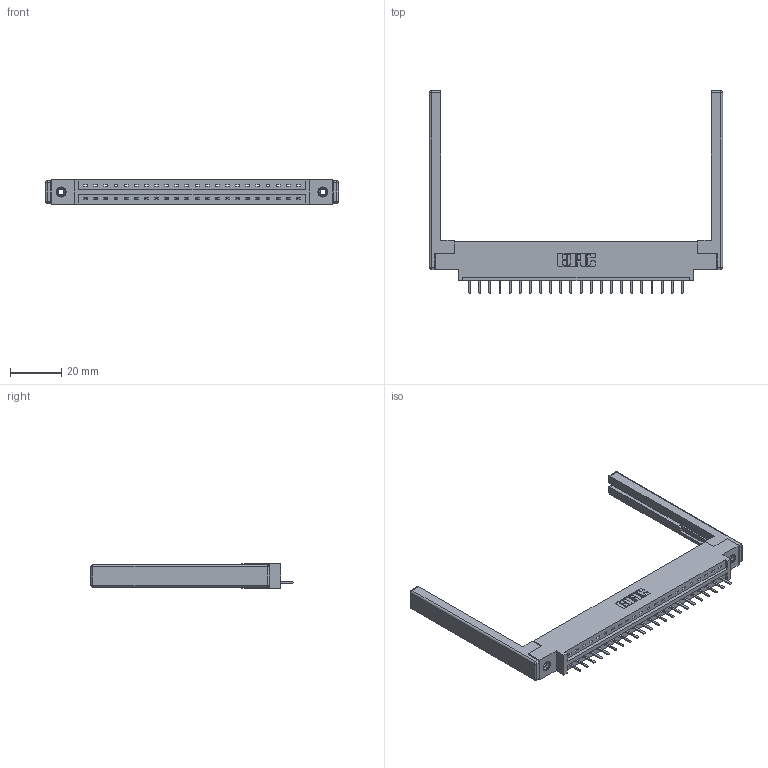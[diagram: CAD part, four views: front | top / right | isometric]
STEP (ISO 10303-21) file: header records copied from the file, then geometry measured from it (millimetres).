
FILE_DESCRIPTION (( 'STEP AP203' ), '1' );
FILE_NAME ('387-022-520-668.STEP', '2019-10-03T00:48:26', ( '' ), ( '' ), 'SwSTEP 2.0', 'SolidWorks 2016', '' );
FILE_SCHEMA (( 'CONFIG_CONTROL_DESIGN' ));
Length unit declared in the file: inch
Products named in the file (5): 387-022-520-668; 337 Part_0.170 Offset - 0.156 Dia-TI; 307-220-068; 345-292-001_345-293-120; 345-250-001_345-250-001-102
Assembly tree (27 placements, depth 2):
  387-022-520-668
    337 Part_0.170 Offset - 0.156 Dia-TI
    345-292-001_345-293-120  x22
    345-250-001_345-250-001-102  x2
    307-220-068  x2
Bounding box: 114.6 x 79.08 x 9.4 mm (x, y, z)
Volume: 15871.4 mm3; surface area: 15713.4 mm2
Topology: 27 solids, 27 shells, 1724 faces, 5025 edges, 3270 vertices
Faces by surface type: plane 1218, cylinder 482, cone 12, sphere 8, torus 4
Entity records: 21946 total; most frequent: CARTESIAN_POINT 3789, ORIENTED_EDGE 3724, DIRECTION 3292, EDGE_CURVE 1862, LINE 1680, VECTOR 1680, VERTEX_POINT 1230, AXIS2_PLACEMENT_3D 806
